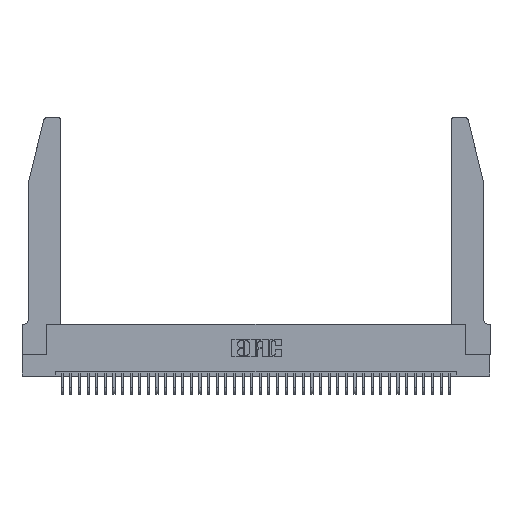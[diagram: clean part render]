
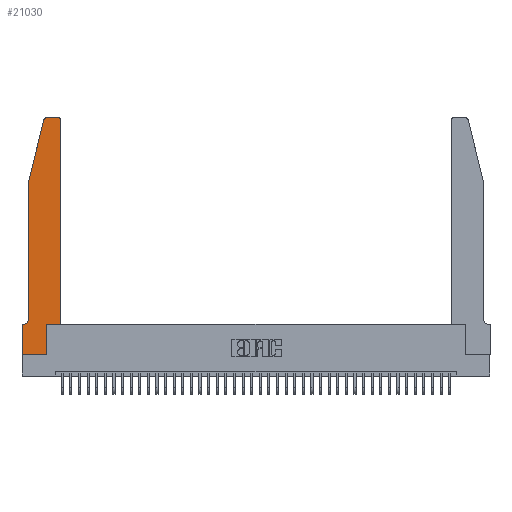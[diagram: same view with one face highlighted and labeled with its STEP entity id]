
A CAD part, top view. The second image highlights one B-rep face of the part: STEP entity #21030.
In plain terms, the highlighted planar face has unit normal (0, 0, 1).
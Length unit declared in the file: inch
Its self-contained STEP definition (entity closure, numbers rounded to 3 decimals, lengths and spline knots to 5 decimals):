
#259 = VERTEX_POINT ( 'NONE', #4306 ) ;
#1439 = CARTESIAN_POINT ( 'NONE',  ( 0., 0., 0.37 ) ) ;
#1773 = EDGE_CURVE ( 'NONE', #30819, #25117, #13656, .T. ) ;
#2239 = LINE ( 'NONE', #29787, #11902 ) ;
#3801 = CARTESIAN_POINT ( 'NONE',  ( 0.4505, 0.35, 0.37 ) ) ;
#3946 = VERTEX_POINT ( 'NONE', #22384 ) ;
#4306 = CARTESIAN_POINT ( 'NONE',  ( 0.0755, 2., 0.37 ) ) ;
#4759 = ORIENTED_EDGE ( 'NONE', *, *, #12437, .T. ) ;
#5157 = ORIENTED_EDGE ( 'NONE', *, *, #39634, .T. ) ;
#6115 = EDGE_CURVE ( 'NONE', #25117, #32611, #34062, .T. ) ;
#6496 = CIRCLE ( 'NONE', #11277, 0.03 ) ;
#6609 = EDGE_CURVE ( 'NONE', #259, #32914, #38633, .T. ) ;
#6794 = EDGE_CURVE ( 'NONE', #40739, #37426, #32580, .T. ) ;
#6897 = CARTESIAN_POINT ( 'NONE',  ( 0.2865, 0., 0.37 ) ) ;
#6963 = EDGE_CURVE ( 'NONE', #37426, #40636, #19851, .T. ) ;
#7892 = VECTOR ( 'NONE', #19630, 39.37008 ) ;
#8018 = AXIS2_PLACEMENT_3D ( 'NONE', #26234, #12815, #28814 ) ;
#8659 = VECTOR ( 'NONE', #9115, 39.37008 ) ;
#8828 = CARTESIAN_POINT ( 'NONE',  ( 0.2865, 0.35, 0.37 ) ) ;
#9115 = DIRECTION ( 'NONE',  ( 0., 1., 0. ) ) ;
#9184 = DIRECTION ( 'NONE',  ( 1., 0., 0. ) ) ;
#9210 = DIRECTION ( 'NONE',  ( 1., 0., 0. ) ) ;
#9237 = DIRECTION ( 'NONE',  ( 1., 0., 0. ) ) ;
#11277 = AXIS2_PLACEMENT_3D ( 'NONE', #19157, #35451, #9184 ) ;
#11814 = CARTESIAN_POINT ( 'NONE',  ( 0.0755, 2., 0.37 ) ) ;
#11902 = VECTOR ( 'NONE', #36437, 39.37008 ) ;
#12223 = ORIENTED_EDGE ( 'NONE', *, *, #6609, .T. ) ;
#12254 = CARTESIAN_POINT ( 'NONE',  ( 0.4505, 2.72, 0.37 ) ) ;
#12268 = CARTESIAN_POINT ( 'NONE',  ( 0.284, 2.72, 0.37 ) ) ;
#12437 = EDGE_CURVE ( 'NONE', #40388, #35340, #38342, .T. ) ;
#12815 = DIRECTION ( 'NONE',  ( 0., 0., 1. ) ) ;
#13049 = CARTESIAN_POINT ( 'NONE',  ( 0.284, 2.75, 0.37 ) ) ;
#13204 = DIRECTION ( 'NONE',  ( -1., 0., 0. ) ) ;
#13333 = CARTESIAN_POINT ( 'NONE',  ( 0.4505, 0.35, 0.37 ) ) ;
#13580 = DIRECTION ( 'NONE',  ( 0., 1., 0. ) ) ;
#13656 = LINE ( 'NONE', #28375, #28875 ) ;
#14306 = CARTESIAN_POINT ( 'NONE',  ( 0.0755, 2., 0.37 ) ) ;
#14489 = CARTESIAN_POINT ( 'NONE',  ( 0., 0.35, 0.37 ) ) ;
#16733 = DIRECTION ( 'NONE',  ( 1., 0., 0. ) ) ;
#17106 = CARTESIAN_POINT ( 'NONE',  ( 0.2605, 2.75, 0.37 ) ) ;
#17258 = EDGE_CURVE ( 'NONE', #35340, #30819, #2239, .T. ) ;
#17567 = ORIENTED_EDGE ( 'NONE', *, *, #6794, .T. ) ;
#17918 = ORIENTED_EDGE ( 'NONE', *, *, #1773, .T. ) ;
#18047 = EDGE_CURVE ( 'NONE', #40636, #259, #25548, .T. ) ;
#18713 = ORIENTED_EDGE ( 'NONE', *, *, #37436, .T. ) ;
#19157 = CARTESIAN_POINT ( 'NONE',  ( 0.4205, 2.72, 0.37 ) ) ;
#19381 = VECTOR ( 'NONE', #23627, 39.37008 ) ;
#19630 = DIRECTION ( 'NONE',  ( -1., 0., 0. ) ) ;
#19851 = CIRCLE ( 'NONE', #33294, 0.03 ) ;
#21030 = ADVANCED_FACE ( 'NONE', ( #22113 ), #38849, .T. ) ;
#21058 = CARTESIAN_POINT ( 'NONE',  ( 0.25487, 2.72718, 0.37 ) ) ;
#22113 = FACE_OUTER_BOUND ( 'NONE', #41227, .T. ) ;
#22213 = CARTESIAN_POINT ( 'NONE',  ( 0.0755, 0.42, 0.37 ) ) ;
#22384 = CARTESIAN_POINT ( 'NONE',  ( 0.4505, 0.35, 0.37 ) ) ;
#22695 = VERTEX_POINT ( 'NONE', #12254 ) ;
#23627 = DIRECTION ( 'NONE',  ( -1., 0., 0. ) ) ;
#24197 = ORIENTED_EDGE ( 'NONE', *, *, #6963, .T. ) ;
#24530 = LINE ( 'NONE', #3801, #39692 ) ;
#25117 = VERTEX_POINT ( 'NONE', #6897 ) ;
#25548 = LINE ( 'NONE', #14306, #38690 ) ;
#25815 = ORIENTED_EDGE ( 'NONE', *, *, #17258, .T. ) ;
#26218 = CARTESIAN_POINT ( 'NONE',  ( 0.0055, 0.42, 0.37 ) ) ;
#26234 = CARTESIAN_POINT ( 'NONE',  ( 0., 0.35, 0.37 ) ) ;
#26354 = ORIENTED_EDGE ( 'NONE', *, *, #28100, .T. ) ;
#28100 = EDGE_CURVE ( 'NONE', #32914, #40388, #33935, .T. ) ;
#28375 = CARTESIAN_POINT ( 'NONE',  ( 0., 0., 0.37 ) ) ;
#28814 = DIRECTION ( 'NONE',  ( 1., 0., 0. ) ) ;
#28822 = VECTOR ( 'NONE', #16733, 39.37008 ) ;
#28875 = VECTOR ( 'NONE', #9210, 39.37008 ) ;
#29003 = VECTOR ( 'NONE', #37731, 39.37008 ) ;
#29556 = CARTESIAN_POINT ( 'NONE',  ( 0.0055, 0.35, 0.37 ) ) ;
#29787 = CARTESIAN_POINT ( 'NONE',  ( 0., 0., 0.37 ) ) ;
#29798 = ORIENTED_EDGE ( 'NONE', *, *, #18047, .T. ) ;
#30260 = ORIENTED_EDGE ( 'NONE', *, *, #6115, .T. ) ;
#30602 = CARTESIAN_POINT ( 'NONE',  ( 0.2865, 0.35, 0.37 ) ) ;
#30819 = VERTEX_POINT ( 'NONE', #1439 ) ;
#32580 = LINE ( 'NONE', #17106, #19381 ) ;
#32611 = VERTEX_POINT ( 'NONE', #30602 ) ;
#32914 = VERTEX_POINT ( 'NONE', #22213 ) ;
#33294 = AXIS2_PLACEMENT_3D ( 'NONE', #12268, #34934, #9237 ) ;
#33935 = CIRCLE ( 'NONE', #40304, 0.07 ) ;
#34032 = EDGE_CURVE ( 'NONE', #32611, #3946, #37435, .T. ) ;
#34062 = LINE ( 'NONE', #8828, #8659 ) ;
#34934 = DIRECTION ( 'NONE',  ( 0., 0., 1. ) ) ;
#35340 = VERTEX_POINT ( 'NONE', #14489 ) ;
#35451 = DIRECTION ( 'NONE',  ( 0., 0., 1. ) ) ;
#36139 = DIRECTION ( 'NONE',  ( 0., 0., -1. ) ) ;
#36437 = DIRECTION ( 'NONE',  ( 0., -1., 0. ) ) ;
#36950 = DIRECTION ( 'NONE',  ( -0.239, -0.971, 0. ) ) ;
#37426 = VERTEX_POINT ( 'NONE', #13049 ) ;
#37435 = LINE ( 'NONE', #13333, #28822 ) ;
#37436 = EDGE_CURVE ( 'NONE', #3946, #22695, #24530, .T. ) ;
#37731 = DIRECTION ( 'NONE',  ( 0., -1., 0. ) ) ;
#38342 = LINE ( 'NONE', #39015, #7892 ) ;
#38633 = LINE ( 'NONE', #11814, #29003 ) ;
#38690 = VECTOR ( 'NONE', #36950, 39.37008 ) ;
#38849 = PLANE ( 'NONE',  #8018 ) ;
#39015 = CARTESIAN_POINT ( 'NONE',  ( 0.0755, 0.35, 0.37 ) ) ;
#39634 = EDGE_CURVE ( 'NONE', #22695, #40739, #6496, .T. ) ;
#39692 = VECTOR ( 'NONE', #13580, 39.37008 ) ;
#40304 = AXIS2_PLACEMENT_3D ( 'NONE', #26218, #36139, #13204 ) ;
#40388 = VERTEX_POINT ( 'NONE', #29556 ) ;
#40587 = CARTESIAN_POINT ( 'NONE',  ( 0.4205, 2.75, 0.37 ) ) ;
#40636 = VERTEX_POINT ( 'NONE', #21058 ) ;
#40739 = VERTEX_POINT ( 'NONE', #40587 ) ;
#41055 = ORIENTED_EDGE ( 'NONE', *, *, #34032, .T. ) ;
#41227 = EDGE_LOOP ( 'NONE', ( #17567, #24197, #29798, #12223, #26354, #4759, #25815, #17918, #30260, #41055, #18713, #5157 ) ) ;
